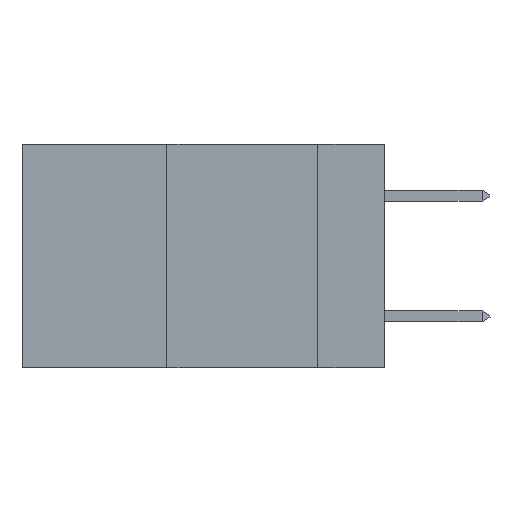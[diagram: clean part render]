
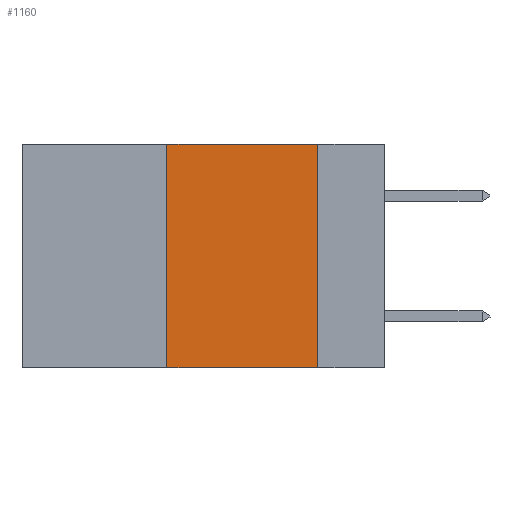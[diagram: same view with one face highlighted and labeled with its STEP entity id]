
A CAD part, left-side view. The second image highlights one B-rep face of the part: STEP entity #1160.
In plain terms, the highlighted planar face has unit normal (-1, 0, 0).
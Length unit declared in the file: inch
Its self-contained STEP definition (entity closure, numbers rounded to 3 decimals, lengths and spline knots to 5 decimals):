
#217 = CARTESIAN_POINT ( 'NONE',  ( 0., 0.11, 0. ) ) ;
#359 = VECTOR ( 'NONE', #7022, 39.37008 ) ;
#1160 = ADVANCED_FACE ( 'NONE', ( #17270 ), #18578, .F. ) ;
#2140 = LINE ( 'NONE', #9814, #5568 ) ;
#2361 = CARTESIAN_POINT ( 'NONE',  ( 0., 0.11, 0. ) ) ;
#2535 = AXIS2_PLACEMENT_3D ( 'NONE', #18697, #18397, #18323 ) ;
#2747 = ORIENTED_EDGE ( 'NONE', *, *, #14030, .F. ) ;
#3390 = VERTEX_POINT ( 'NONE', #17477 ) ;
#4525 = ORIENTED_EDGE ( 'NONE', *, *, #9180, .T. ) ;
#5568 = VECTOR ( 'NONE', #15611, 39.37008 ) ;
#5809 = CARTESIAN_POINT ( 'NONE',  ( 0., 0.6, 0. ) ) ;
#5908 = CARTESIAN_POINT ( 'NONE',  ( 0., 0.36, 0. ) ) ;
#6675 = LINE ( 'NONE', #2361, #7608 ) ;
#7022 = DIRECTION ( 'NONE',  ( 0., -1., 0. ) ) ;
#7277 = DIRECTION ( 'NONE',  ( 0., -1., 0. ) ) ;
#7608 = VECTOR ( 'NONE', #12554, 39.37008 ) ;
#7702 = EDGE_CURVE ( 'NONE', #18711, #10333, #6675, .T. ) ;
#8235 = LINE ( 'NONE', #15711, #359 ) ;
#8846 = LINE ( 'NONE', #5809, #16064 ) ;
#9180 = EDGE_CURVE ( 'NONE', #3390, #10333, #8235, .T. ) ;
#9814 = CARTESIAN_POINT ( 'NONE',  ( 0., 0.36, 0. ) ) ;
#10333 = VERTEX_POINT ( 'NONE', #17012 ) ;
#10384 = EDGE_LOOP ( 'NONE', ( #14369, #16120, #2747, #4525 ) ) ;
#11215 = EDGE_CURVE ( 'NONE', #15460, #18711, #8846, .T. ) ;
#12554 = DIRECTION ( 'NONE',  ( 0., 0., -1. ) ) ;
#14030 = EDGE_CURVE ( 'NONE', #3390, #15460, #2140, .T. ) ;
#14369 = ORIENTED_EDGE ( 'NONE', *, *, #7702, .F. ) ;
#15460 = VERTEX_POINT ( 'NONE', #5908 ) ;
#15611 = DIRECTION ( 'NONE',  ( 0., 0., 1. ) ) ;
#15711 = CARTESIAN_POINT ( 'NONE',  ( 0., 0.6, -0.37 ) ) ;
#16064 = VECTOR ( 'NONE', #7277, 39.37008 ) ;
#16120 = ORIENTED_EDGE ( 'NONE', *, *, #11215, .F. ) ;
#17012 = CARTESIAN_POINT ( 'NONE',  ( 0., 0.11, -0.37 ) ) ;
#17270 = FACE_OUTER_BOUND ( 'NONE', #10384, .T. ) ;
#17477 = CARTESIAN_POINT ( 'NONE',  ( 0., 0.36, -0.37 ) ) ;
#18323 = DIRECTION ( 'NONE',  ( 0., 0., -1. ) ) ;
#18397 = DIRECTION ( 'NONE',  ( 1., 0., 0. ) ) ;
#18578 = PLANE ( 'NONE',  #2535 ) ;
#18697 = CARTESIAN_POINT ( 'NONE',  ( 0., 0.6, 0. ) ) ;
#18711 = VERTEX_POINT ( 'NONE', #217 ) ;
